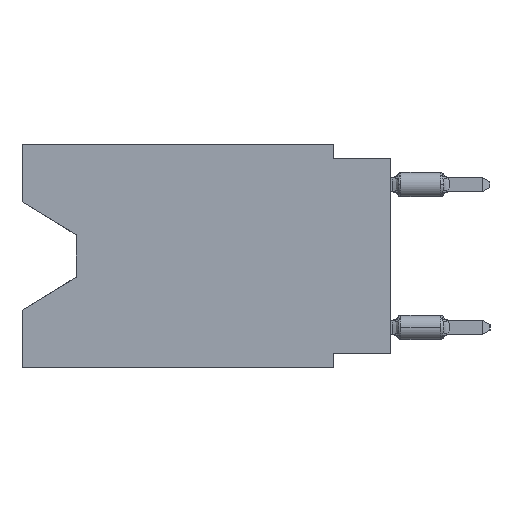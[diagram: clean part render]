
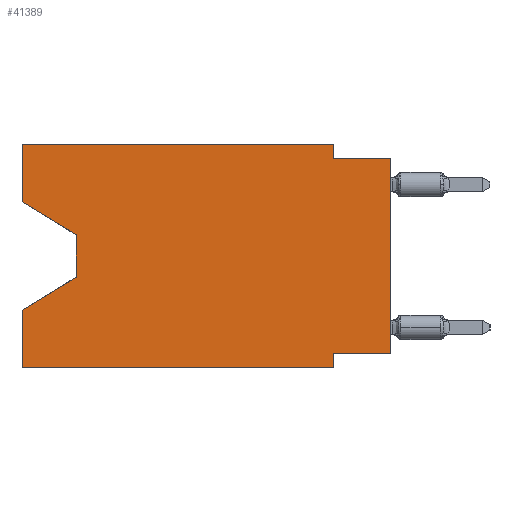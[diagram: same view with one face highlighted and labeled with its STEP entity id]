
A CAD part, left-side view. The second image highlights one B-rep face of the part: STEP entity #41389.
In plain terms, the highlighted planar face has unit normal (-1, 0, 0).
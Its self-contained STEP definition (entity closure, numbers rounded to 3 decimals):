
#1628 = DIRECTION ( 'NONE',  ( 0., 0., 1. ) ) ;
#2165 = VECTOR ( 'NONE', #5521, 1000. ) ;
#2483 = EDGE_CURVE ( 'NONE', #34900, #58086, #51097, .T. ) ;
#2537 = EDGE_CURVE ( 'NONE', #48437, #48213, #50167, .T. ) ;
#2589 = EDGE_CURVE ( 'NONE', #34900, #12231, #57812, .T. ) ;
#2775 = CARTESIAN_POINT ( 'NONE',  ( 0., 16.383, -9.906 ) ) ;
#3298 = DIRECTION ( 'NONE',  ( 0., -1., 0. ) ) ;
#3929 = EDGE_CURVE ( 'NONE', #48437, #32664, #28941, .T. ) ;
#5490 = DIRECTION ( 'NONE',  ( 0., 0., -1. ) ) ;
#5521 = DIRECTION ( 'NONE',  ( 0., 0., 1. ) ) ;
#6216 = DIRECTION ( 'NONE',  ( 0., 1., 0. ) ) ;
#6813 = CARTESIAN_POINT ( 'NONE',  ( 0., 0., -0.635 ) ) ;
#8771 = VECTOR ( 'NONE', #30901, 1000. ) ;
#10472 = ORIENTED_EDGE ( 'NONE', *, *, #11275, .T. ) ;
#10479 = EDGE_CURVE ( 'NONE', #48213, #12231, #49751, .T. ) ;
#10687 = LINE ( 'NONE', #25764, #8771 ) ;
#11275 = EDGE_CURVE ( 'NONE', #35338, #27883, #10687, .T. ) ;
#11578 = ORIENTED_EDGE ( 'NONE', *, *, #44493, .F. ) ;
#12231 = VERTEX_POINT ( 'NONE', #56706 ) ;
#12568 = LINE ( 'NONE', #6813, #24268 ) ;
#13075 = ORIENTED_EDGE ( 'NONE', *, *, #2537, .F. ) ;
#14089 = CARTESIAN_POINT ( 'NONE',  ( 0., 13.97, -4.013 ) ) ;
#14216 = CARTESIAN_POINT ( 'NONE',  ( 0., 16.383, 0. ) ) ;
#14538 = VERTEX_POINT ( 'NONE', #22602 ) ;
#15081 = LINE ( 'NONE', #43969, #54748 ) ;
#15153 = DIRECTION ( 'NONE',  ( 0., 0., -1. ) ) ;
#15818 = DIRECTION ( 'NONE',  ( 0., 0., 1. ) ) ;
#16499 = CARTESIAN_POINT ( 'NONE',  ( 0., 16.383, -2.546 ) ) ;
#16699 = LINE ( 'NONE', #22459, #21990 ) ;
#17417 = VECTOR ( 'NONE', #6216, 1000. ) ;
#18022 = EDGE_CURVE ( 'NONE', #31031, #44028, #39559, .T. ) ;
#19241 = ORIENTED_EDGE ( 'NONE', *, *, #36041, .T. ) ;
#21680 = ORIENTED_EDGE ( 'NONE', *, *, #2589, .T. ) ;
#21990 = VECTOR ( 'NONE', #1628, 1000. ) ;
#22459 = CARTESIAN_POINT ( 'NONE',  ( 0., 16.383, 0. ) ) ;
#22602 = CARTESIAN_POINT ( 'NONE',  ( 0., 16.383, 0. ) ) ;
#23490 = ORIENTED_EDGE ( 'NONE', *, *, #3929, .T. ) ;
#23645 = CARTESIAN_POINT ( 'NONE',  ( 0., 2.54, 0. ) ) ;
#23683 = ORIENTED_EDGE ( 'NONE', *, *, #2483, .F. ) ;
#23845 = FACE_OUTER_BOUND ( 'NONE', #62963, .T. ) ;
#24268 = VECTOR ( 'NONE', #45311, 1000. ) ;
#25390 = EDGE_CURVE ( 'NONE', #44028, #32664, #12568, .T. ) ;
#25764 = CARTESIAN_POINT ( 'NONE',  ( 0., 16.383, -2.546 ) ) ;
#27883 = VERTEX_POINT ( 'NONE', #35477 ) ;
#28666 = CARTESIAN_POINT ( 'NONE',  ( 0., 2.54, -9.271 ) ) ;
#28941 = LINE ( 'NONE', #34072, #2165 ) ;
#30331 = ORIENTED_EDGE ( 'NONE', *, *, #25390, .F. ) ;
#30901 = DIRECTION ( 'NONE',  ( 0., -0.855, -0.519 ) ) ;
#31031 = VERTEX_POINT ( 'NONE', #23645 ) ;
#32664 = VERTEX_POINT ( 'NONE', #35029 ) ;
#32972 = VERTEX_POINT ( 'NONE', #48127 ) ;
#33365 = CARTESIAN_POINT ( 'NONE',  ( 0., 16.383, 0. ) ) ;
#34072 = CARTESIAN_POINT ( 'NONE',  ( 0., 0., 0. ) ) ;
#34406 = ORIENTED_EDGE ( 'NONE', *, *, #10479, .F. ) ;
#34829 = VECTOR ( 'NONE', #3298, 1000. ) ;
#34900 = VERTEX_POINT ( 'NONE', #2775 ) ;
#34989 = CARTESIAN_POINT ( 'NONE',  ( 0., 2.54, -9.906 ) ) ;
#35029 = CARTESIAN_POINT ( 'NONE',  ( 0., 0., -0.635 ) ) ;
#35338 = VERTEX_POINT ( 'NONE', #16499 ) ;
#35477 = CARTESIAN_POINT ( 'NONE',  ( 0., 13.97, -4.013 ) ) ;
#36041 = EDGE_CURVE ( 'NONE', #32972, #58086, #15081, .T. ) ;
#36261 = ORIENTED_EDGE ( 'NONE', *, *, #56645, .T. ) ;
#38611 = DIRECTION ( 'NONE',  ( 0., 0., -1. ) ) ;
#39256 = CARTESIAN_POINT ( 'NONE',  ( 0., 0., -9.271 ) ) ;
#39559 = LINE ( 'NONE', #59141, #43216 ) ;
#40465 = VECTOR ( 'NONE', #53258, 1000. ) ;
#40607 = VECTOR ( 'NONE', #5490, 1000. ) ;
#40833 = CARTESIAN_POINT ( 'NONE',  ( 0., 16.383, 0. ) ) ;
#41126 = ORIENTED_EDGE ( 'NONE', *, *, #56449, .F. ) ;
#41389 = ADVANCED_FACE ( 'NONE', ( #23845 ), #43413, .F. ) ;
#43216 = VECTOR ( 'NONE', #15153, 1000. ) ;
#43294 = LINE ( 'NONE', #14089, #40465 ) ;
#43413 = PLANE ( 'NONE',  #52140 ) ;
#43969 = CARTESIAN_POINT ( 'NONE',  ( 0., 13.97, -5.893 ) ) ;
#44028 = VERTEX_POINT ( 'NONE', #55913 ) ;
#44493 = EDGE_CURVE ( 'NONE', #14538, #31031, #48768, .T. ) ;
#45311 = DIRECTION ( 'NONE',  ( 0., -1., 0. ) ) ;
#47108 = VECTOR ( 'NONE', #15818, 1000. ) ;
#48127 = CARTESIAN_POINT ( 'NONE',  ( 0., 13.97, -5.893 ) ) ;
#48183 = CARTESIAN_POINT ( 'NONE',  ( 0., 16.383, -9.906 ) ) ;
#48213 = VERTEX_POINT ( 'NONE', #28666 ) ;
#48437 = VERTEX_POINT ( 'NONE', #39256 ) ;
#48768 = LINE ( 'NONE', #33365, #61624 ) ;
#49751 = LINE ( 'NONE', #34989, #40607 ) ;
#50167 = LINE ( 'NONE', #55605, #17417 ) ;
#51097 = LINE ( 'NONE', #40833, #47108 ) ;
#52140 = AXIS2_PLACEMENT_3D ( 'NONE', #14216, #62993, #38611 ) ;
#53258 = DIRECTION ( 'NONE',  ( 0., 0., -1. ) ) ;
#54748 = VECTOR ( 'NONE', #63225, 1000. ) ;
#54854 = CARTESIAN_POINT ( 'NONE',  ( 0., 16.383, -7.36 ) ) ;
#55605 = CARTESIAN_POINT ( 'NONE',  ( 0., 0., -9.271 ) ) ;
#55913 = CARTESIAN_POINT ( 'NONE',  ( 0., 2.54, -0.635 ) ) ;
#56449 = EDGE_CURVE ( 'NONE', #35338, #14538, #16699, .T. ) ;
#56645 = EDGE_CURVE ( 'NONE', #27883, #32972, #43294, .T. ) ;
#56706 = CARTESIAN_POINT ( 'NONE',  ( 0., 2.54, -9.906 ) ) ;
#57812 = LINE ( 'NONE', #48183, #34829 ) ;
#58086 = VERTEX_POINT ( 'NONE', #54854 ) ;
#58715 = DIRECTION ( 'NONE',  ( 0., -1., 0. ) ) ;
#59141 = CARTESIAN_POINT ( 'NONE',  ( 0., 2.54, 0. ) ) ;
#59887 = ORIENTED_EDGE ( 'NONE', *, *, #18022, .F. ) ;
#61624 = VECTOR ( 'NONE', #58715, 1000. ) ;
#62963 = EDGE_LOOP ( 'NONE', ( #10472, #36261, #19241, #23683, #21680, #34406, #13075, #23490, #30331, #59887, #11578, #41126 ) ) ;
#62993 = DIRECTION ( 'NONE',  ( 1., 0., 0. ) ) ;
#63225 = DIRECTION ( 'NONE',  ( 0., 0.855, -0.519 ) ) ;
